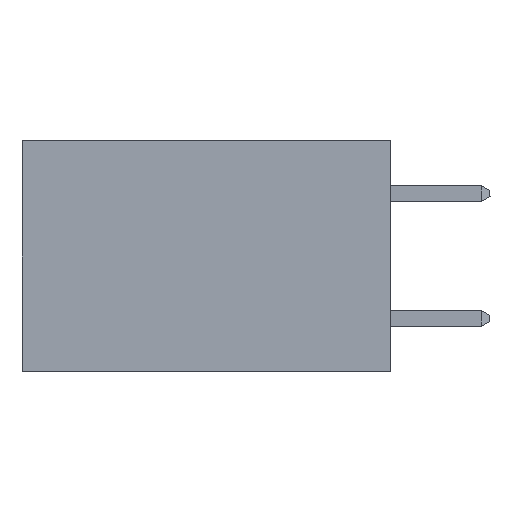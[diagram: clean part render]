
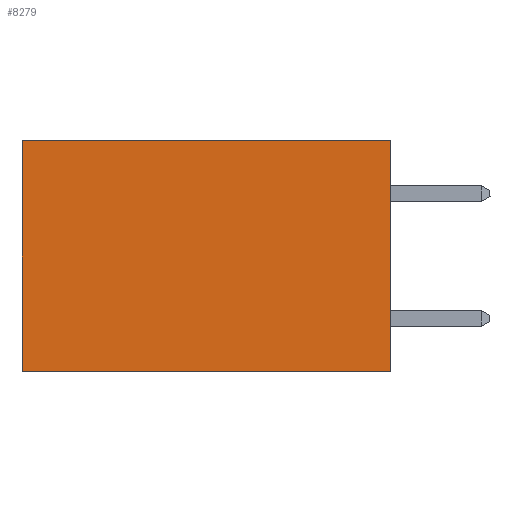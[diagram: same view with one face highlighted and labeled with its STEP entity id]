
A CAD part, left-side view. The second image highlights one B-rep face of the part: STEP entity #8279.
In plain terms, the highlighted planar face has unit normal (-1, 0, 0).
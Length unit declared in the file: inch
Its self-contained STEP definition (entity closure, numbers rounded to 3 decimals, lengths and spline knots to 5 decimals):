
#184 = VECTOR ( 'NONE', #7823, 39.37008 ) ;
#240 = CARTESIAN_POINT ( 'NONE',  ( 0.277, 0.59, 0. ) ) ;
#3159 = VERTEX_POINT ( 'NONE', #240 ) ;
#3558 = VERTEX_POINT ( 'NONE', #18922 ) ;
#4196 = VERTEX_POINT ( 'NONE', #10611 ) ;
#5252 = CARTESIAN_POINT ( 'NONE',  ( 0.277, 0., 0. ) ) ;
#5471 = ORIENTED_EDGE ( 'NONE', *, *, #29239, .T. ) ;
#6032 = EDGE_CURVE ( 'NONE', #3159, #4196, #21577, .T. ) ;
#7823 = DIRECTION ( 'NONE',  ( 0., 1., 0. ) ) ;
#8279 = ADVANCED_FACE ( 'NONE', ( #16404 ), #21148, .F. ) ;
#9593 = DIRECTION ( 'NONE',  ( 0., 0., -1. ) ) ;
#10611 = CARTESIAN_POINT ( 'NONE',  ( 0.277, 0.59, -0.37 ) ) ;
#11762 = CARTESIAN_POINT ( 'NONE',  ( 0.277, 0., -0.37 ) ) ;
#12017 = CARTESIAN_POINT ( 'NONE',  ( 0.277, 0., -0.37 ) ) ;
#13720 = DIRECTION ( 'NONE',  ( 1., 0., 0. ) ) ;
#13753 = LINE ( 'NONE', #11762, #21274 ) ;
#15668 = VECTOR ( 'NONE', #19774, 39.37008 ) ;
#16404 = FACE_OUTER_BOUND ( 'NONE', #22489, .T. ) ;
#18040 = VECTOR ( 'NONE', #9593, 39.37008 ) ;
#18922 = CARTESIAN_POINT ( 'NONE',  ( 0.277, 0., -0.37 ) ) ;
#19774 = DIRECTION ( 'NONE',  ( 0., 0., -1. ) ) ;
#20088 = CARTESIAN_POINT ( 'NONE',  ( 0.277, 0.59, -0.37 ) ) ;
#20276 = LINE ( 'NONE', #5252, #184 ) ;
#21148 = PLANE ( 'NONE',  #22705 ) ;
#21274 = VECTOR ( 'NONE', #29172, 39.37008 ) ;
#21505 = ORIENTED_EDGE ( 'NONE', *, *, #6032, .T. ) ;
#21577 = LINE ( 'NONE', #20088, #15668 ) ;
#22489 = EDGE_LOOP ( 'NONE', ( #21505, #27361, #22903, #5471 ) ) ;
#22705 = AXIS2_PLACEMENT_3D ( 'NONE', #26196, #13720, #31096 ) ;
#22903 = ORIENTED_EDGE ( 'NONE', *, *, #27581, .F. ) ;
#25187 = CARTESIAN_POINT ( 'NONE',  ( 0.277, 0., 0. ) ) ;
#26194 = EDGE_CURVE ( 'NONE', #3558, #4196, #13753, .T. ) ;
#26196 = CARTESIAN_POINT ( 'NONE',  ( 0.277, 0., -0.37 ) ) ;
#27361 = ORIENTED_EDGE ( 'NONE', *, *, #26194, .F. ) ;
#27581 = EDGE_CURVE ( 'NONE', #29985, #3558, #31142, .T. ) ;
#29172 = DIRECTION ( 'NONE',  ( 0., 1., 0. ) ) ;
#29239 = EDGE_CURVE ( 'NONE', #29985, #3159, #20276, .T. ) ;
#29985 = VERTEX_POINT ( 'NONE', #25187 ) ;
#31096 = DIRECTION ( 'NONE',  ( 0., 0., -1. ) ) ;
#31142 = LINE ( 'NONE', #12017, #18040 ) ;
